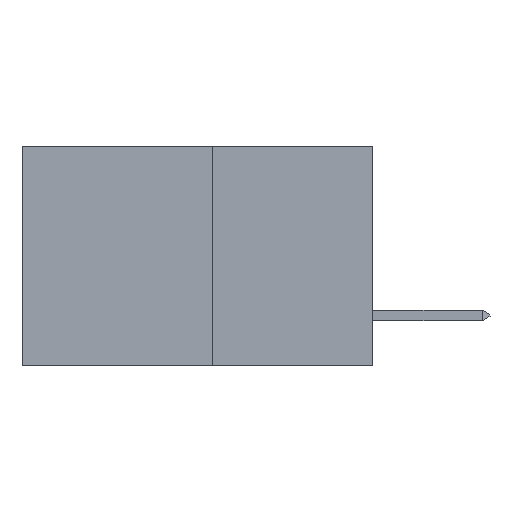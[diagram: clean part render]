
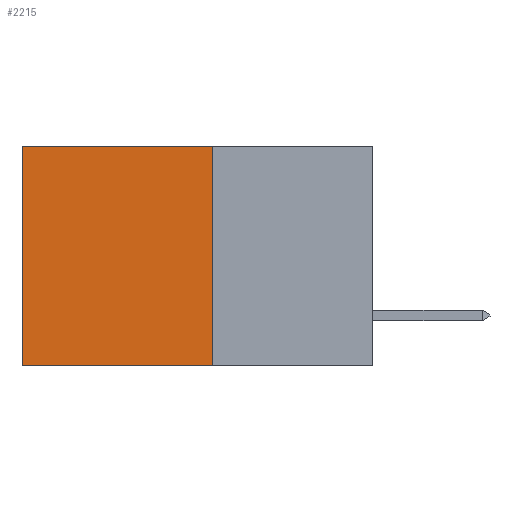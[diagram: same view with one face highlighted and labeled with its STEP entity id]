
A CAD part, left-side view. The second image highlights one B-rep face of the part: STEP entity #2215.
In plain terms, the highlighted planar face has unit normal (-1, 0, 0).
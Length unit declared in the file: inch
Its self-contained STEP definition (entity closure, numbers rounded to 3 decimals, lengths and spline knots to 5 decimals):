
#937 = CARTESIAN_POINT ( 'NONE',  ( 0.277, 0.27, 0. ) ) ;
#1074 = DIRECTION ( 'NONE',  ( 0., 1., 0. ) ) ;
#1456 = LINE ( 'NONE', #937, #11096 ) ;
#1617 = DIRECTION ( 'NONE',  ( 0., 0., -1. ) ) ;
#2125 = VECTOR ( 'NONE', #8792, 39.37008 ) ;
#2215 = ADVANCED_FACE ( 'NONE', ( #4006 ), #9086, .F. ) ;
#2322 = VECTOR ( 'NONE', #1074, 39.37008 ) ;
#2371 = CARTESIAN_POINT ( 'NONE',  ( 0.277, 0.27, -0.37 ) ) ;
#2428 = CARTESIAN_POINT ( 'NONE',  ( 0.277, 0.59, -0.37 ) ) ;
#2583 = VERTEX_POINT ( 'NONE', #9200 ) ;
#2600 = CARTESIAN_POINT ( 'NONE',  ( 0.277, 0.59, 0. ) ) ;
#3218 = AXIS2_PLACEMENT_3D ( 'NONE', #4034, #7679, #1617 ) ;
#4006 = FACE_OUTER_BOUND ( 'NONE', #10817, .T. ) ;
#4034 = CARTESIAN_POINT ( 'NONE',  ( 0.277, 0.27, -0.37 ) ) ;
#4155 = LINE ( 'NONE', #11067, #8995 ) ;
#4394 = EDGE_CURVE ( 'NONE', #6081, #7496, #6668, .T. ) ;
#4663 = ORIENTED_EDGE ( 'NONE', *, *, #7768, .T. ) ;
#4763 = ORIENTED_EDGE ( 'NONE', *, *, #11243, .F. ) ;
#5620 = DIRECTION ( 'NONE',  ( 0., 0., -1. ) ) ;
#6081 = VERTEX_POINT ( 'NONE', #2600 ) ;
#6668 = LINE ( 'NONE', #2428, #2125 ) ;
#6831 = EDGE_CURVE ( 'NONE', #11493, #7496, #7457, .T. ) ;
#7312 = DIRECTION ( 'NONE',  ( 0., 1., 0. ) ) ;
#7450 = CARTESIAN_POINT ( 'NONE',  ( 0.277, 0.27, -0.37 ) ) ;
#7457 = LINE ( 'NONE', #7450, #2322 ) ;
#7496 = VERTEX_POINT ( 'NONE', #7648 ) ;
#7648 = CARTESIAN_POINT ( 'NONE',  ( 0.277, 0.59, -0.37 ) ) ;
#7679 = DIRECTION ( 'NONE',  ( 1., 0., 0. ) ) ;
#7768 = EDGE_CURVE ( 'NONE', #2583, #6081, #1456, .T. ) ;
#8792 = DIRECTION ( 'NONE',  ( 0., 0., -1. ) ) ;
#8995 = VECTOR ( 'NONE', #5620, 39.37008 ) ;
#9086 = PLANE ( 'NONE',  #3218 ) ;
#9200 = CARTESIAN_POINT ( 'NONE',  ( 0.277, 0.27, 0. ) ) ;
#9829 = ORIENTED_EDGE ( 'NONE', *, *, #4394, .T. ) ;
#10817 = EDGE_LOOP ( 'NONE', ( #9829, #11524, #4763, #4663 ) ) ;
#11067 = CARTESIAN_POINT ( 'NONE',  ( 0.277, 0.27, -0.37 ) ) ;
#11096 = VECTOR ( 'NONE', #7312, 39.37008 ) ;
#11243 = EDGE_CURVE ( 'NONE', #2583, #11493, #4155, .T. ) ;
#11493 = VERTEX_POINT ( 'NONE', #2371 ) ;
#11524 = ORIENTED_EDGE ( 'NONE', *, *, #6831, .F. ) ;
